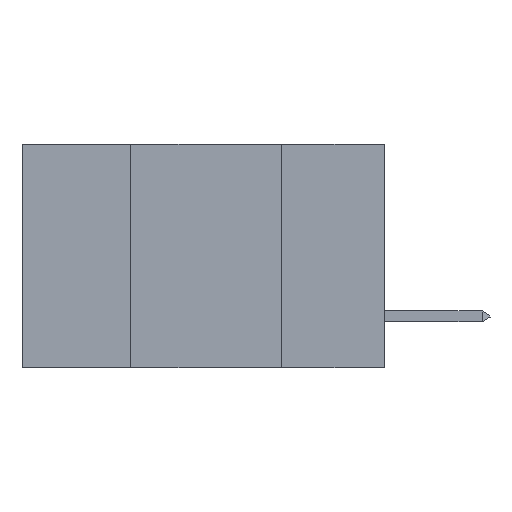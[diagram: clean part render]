
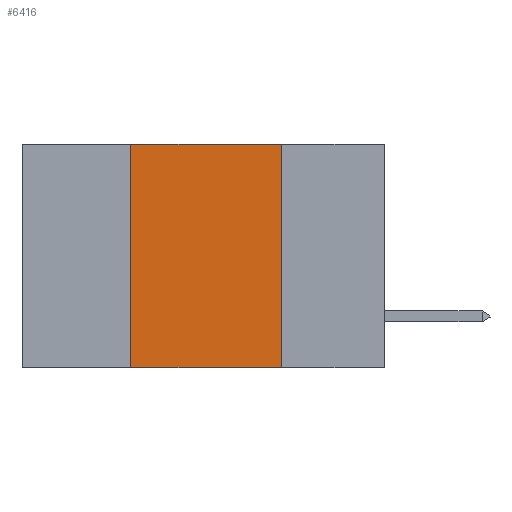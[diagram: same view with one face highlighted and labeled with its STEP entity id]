
A CAD part, left-side view. The second image highlights one B-rep face of the part: STEP entity #6416.
In plain terms, the highlighted planar face has unit normal (-1, 0, 0).
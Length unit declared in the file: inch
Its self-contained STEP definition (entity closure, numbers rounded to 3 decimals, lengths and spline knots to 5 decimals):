
#596 = VECTOR ( 'NONE', #12528, 39.37008 ) ;
#702 = AXIS2_PLACEMENT_3D ( 'NONE', #13954, #9494, #3681 ) ;
#1264 = EDGE_CURVE ( 'NONE', #9464, #15053, #13026, .T. ) ;
#1440 = CARTESIAN_POINT ( 'NONE',  ( 0., 0.42, 0. ) ) ;
#1882 = CARTESIAN_POINT ( 'NONE',  ( 0., 0.6, -0.37 ) ) ;
#2167 = ORIENTED_EDGE ( 'NONE', *, *, #12175, .F. ) ;
#2427 = ORIENTED_EDGE ( 'NONE', *, *, #1264, .F. ) ;
#2660 = DIRECTION ( 'NONE',  ( 0., 0., 1. ) ) ;
#2886 = LINE ( 'NONE', #3837, #14043 ) ;
#3681 = DIRECTION ( 'NONE',  ( 0., 0., -1. ) ) ;
#3837 = CARTESIAN_POINT ( 'NONE',  ( 0., 0.17, 0. ) ) ;
#4063 = LINE ( 'NONE', #1882, #596 ) ;
#5042 = CARTESIAN_POINT ( 'NONE',  ( 0., 0.42, 0. ) ) ;
#6100 = CARTESIAN_POINT ( 'NONE',  ( 0., 0.6, 0. ) ) ;
#6220 = DIRECTION ( 'NONE',  ( 0., 0., -1. ) ) ;
#6402 = ORIENTED_EDGE ( 'NONE', *, *, #12200, .F. ) ;
#6416 = ADVANCED_FACE ( 'NONE', ( #11823 ), #10579, .F. ) ;
#6620 = VERTEX_POINT ( 'NONE', #12571 ) ;
#7162 = VECTOR ( 'NONE', #12038, 39.37008 ) ;
#7172 = CARTESIAN_POINT ( 'NONE',  ( 0., 0.17, 0. ) ) ;
#9464 = VERTEX_POINT ( 'NONE', #1440 ) ;
#9494 = DIRECTION ( 'NONE',  ( 1., 0., 0. ) ) ;
#10124 = VERTEX_POINT ( 'NONE', #12511 ) ;
#10368 = VECTOR ( 'NONE', #2660, 39.37008 ) ;
#10579 = PLANE ( 'NONE',  #702 ) ;
#10951 = LINE ( 'NONE', #5042, #10368 ) ;
#11823 = FACE_OUTER_BOUND ( 'NONE', #13537, .T. ) ;
#12038 = DIRECTION ( 'NONE',  ( 0., -1., 0. ) ) ;
#12175 = EDGE_CURVE ( 'NONE', #15053, #6620, #2886, .T. ) ;
#12200 = EDGE_CURVE ( 'NONE', #10124, #9464, #10951, .T. ) ;
#12511 = CARTESIAN_POINT ( 'NONE',  ( 0., 0.42, -0.37 ) ) ;
#12528 = DIRECTION ( 'NONE',  ( 0., -1., 0. ) ) ;
#12571 = CARTESIAN_POINT ( 'NONE',  ( 0., 0.17, -0.37 ) ) ;
#13026 = LINE ( 'NONE', #6100, #7162 ) ;
#13537 = EDGE_LOOP ( 'NONE', ( #2167, #2427, #6402, #14084 ) ) ;
#13954 = CARTESIAN_POINT ( 'NONE',  ( 0., 0.6, 0. ) ) ;
#14043 = VECTOR ( 'NONE', #6220, 39.37008 ) ;
#14084 = ORIENTED_EDGE ( 'NONE', *, *, #15180, .T. ) ;
#15053 = VERTEX_POINT ( 'NONE', #7172 ) ;
#15180 = EDGE_CURVE ( 'NONE', #10124, #6620, #4063, .T. ) ;
